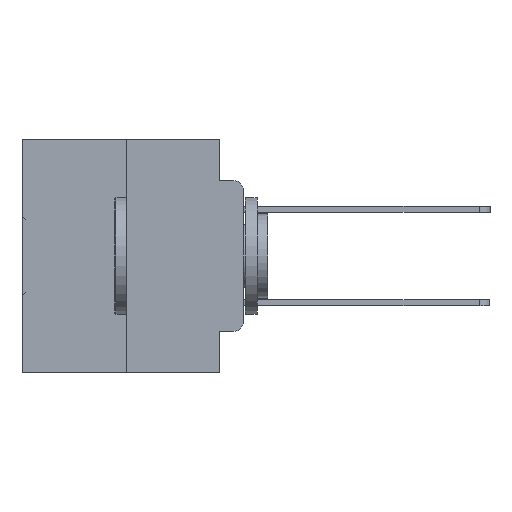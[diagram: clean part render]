
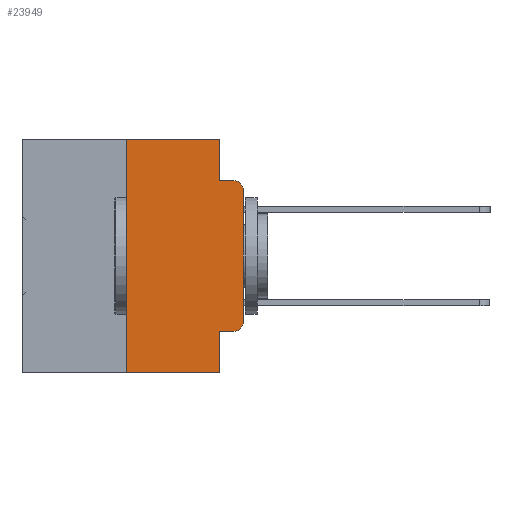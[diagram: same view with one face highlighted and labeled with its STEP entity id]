
A CAD part, left-side view. The second image highlights one B-rep face of the part: STEP entity #23949.
In plain terms, the highlighted planar face has unit normal (-1, 0, 0).
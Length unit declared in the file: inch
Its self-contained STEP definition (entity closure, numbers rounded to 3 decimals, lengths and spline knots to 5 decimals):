
#451 = CARTESIAN_POINT ( 'NONE',  ( 0., 0.25, 0. ) ) ;
#971 = CARTESIAN_POINT ( 'NONE',  ( 0., 0., 0. ) ) ;
#1278 = CARTESIAN_POINT ( 'NONE',  ( 0., 0.473, -0.5 ) ) ;
#2101 = CARTESIAN_POINT ( 'NONE',  ( 0., 0.051, 0. ) ) ;
#2289 = AXIS2_PLACEMENT_3D ( 'NONE', #9709, #33688, #33618 ) ;
#3252 = VERTEX_POINT ( 'NONE', #20303 ) ;
#3353 = EDGE_CURVE ( 'NONE', #3252, #34849, #17456, .T. ) ;
#3633 = VERTEX_POINT ( 'NONE', #451 ) ;
#3754 = DIRECTION ( 'NONE',  ( 0., 0., 1. ) ) ;
#3814 = EDGE_CURVE ( 'NONE', #25659, #6525, #9236, .T. ) ;
#3856 = CARTESIAN_POINT ( 'NONE',  ( 0., 0.473, 0. ) ) ;
#3918 = VECTOR ( 'NONE', #20475, 39.37008 ) ;
#4175 = LINE ( 'NONE', #971, #11537 ) ;
#4646 = ORIENTED_EDGE ( 'NONE', *, *, #3814, .T. ) ;
#4874 = DIRECTION ( 'NONE',  ( 0., 0., -1. ) ) ;
#4879 = VERTEX_POINT ( 'NONE', #22908 ) ;
#5162 = LINE ( 'NONE', #27346, #18997 ) ;
#6348 = EDGE_CURVE ( 'NONE', #4879, #3633, #18604, .T. ) ;
#6525 = VERTEX_POINT ( 'NONE', #30867 ) ;
#6730 = DIRECTION ( 'NONE',  ( 0., -1., 0. ) ) ;
#6808 = DIRECTION ( 'NONE',  ( 0., -1., 0. ) ) ;
#7438 = CARTESIAN_POINT ( 'NONE',  ( 0., 0.051, 0. ) ) ;
#7561 = DIRECTION ( 'NONE',  ( 0., 0., -1. ) ) ;
#7734 = CARTESIAN_POINT ( 'NONE',  ( 0., 0.051, -0.0885 ) ) ;
#7760 = EDGE_CURVE ( 'NONE', #4879, #29713, #17618, .T. ) ;
#8117 = ORIENTED_EDGE ( 'NONE', *, *, #13785, .F. ) ;
#8230 = CARTESIAN_POINT ( 'NONE',  ( 0., 0.473, 0. ) ) ;
#9067 = VECTOR ( 'NONE', #6730, 39.37008 ) ;
#9236 = CIRCLE ( 'NONE', #18238, 0.02 ) ;
#9709 = CARTESIAN_POINT ( 'NONE',  ( 0., 0.02, -0.3915 ) ) ;
#9847 = ORIENTED_EDGE ( 'NONE', *, *, #22464, .F. ) ;
#10311 = ORIENTED_EDGE ( 'NONE', *, *, #3353, .T. ) ;
#10497 = CARTESIAN_POINT ( 'NONE',  ( 0., 0., -0.3915 ) ) ;
#10728 = VECTOR ( 'NONE', #4874, 39.37008 ) ;
#11012 = DIRECTION ( 'NONE',  ( 0., 0., -1. ) ) ;
#11384 = CARTESIAN_POINT ( 'NONE',  ( 0., 0.051, 0. ) ) ;
#11405 = DIRECTION ( 'NONE',  ( 0., 0., -1. ) ) ;
#11452 = DIRECTION ( 'NONE',  ( -1., 0., 0. ) ) ;
#11457 = CARTESIAN_POINT ( 'NONE',  ( 0., 0.02, -0.1085 ) ) ;
#11537 = VECTOR ( 'NONE', #3754, 39.37008 ) ;
#11588 = ORIENTED_EDGE ( 'NONE', *, *, #6348, .F. ) ;
#11998 = VECTOR ( 'NONE', #7561, 39.37008 ) ;
#12059 = AXIS2_PLACEMENT_3D ( 'NONE', #8230, #27543, #11012 ) ;
#12617 = EDGE_CURVE ( 'NONE', #27718, #3252, #5162, .T. ) ;
#13785 = EDGE_CURVE ( 'NONE', #29463, #30838, #26687, .T. ) ;
#14989 = CARTESIAN_POINT ( 'NONE',  ( 0., 0.051, -0.5 ) ) ;
#15268 = LINE ( 'NONE', #24024, #22658 ) ;
#17016 = CARTESIAN_POINT ( 'NONE',  ( 0., 0.051, -0.4115 ) ) ;
#17244 = LINE ( 'NONE', #3856, #9067 ) ;
#17456 = CIRCLE ( 'NONE', #2289, 0.02 ) ;
#17618 = LINE ( 'NONE', #1278, #29750 ) ;
#18238 = AXIS2_PLACEMENT_3D ( 'NONE', #11457, #11452, #11405 ) ;
#18467 = ORIENTED_EDGE ( 'NONE', *, *, #24202, .T. ) ;
#18604 = LINE ( 'NONE', #28901, #3918 ) ;
#18997 = VECTOR ( 'NONE', #24615, 39.37008 ) ;
#19333 = EDGE_CURVE ( 'NONE', #30838, #6525, #15268, .T. ) ;
#19432 = CARTESIAN_POINT ( 'NONE',  ( 0., 0., -0.1085 ) ) ;
#20303 = CARTESIAN_POINT ( 'NONE',  ( 0., 0.02, -0.4115 ) ) ;
#20475 = DIRECTION ( 'NONE',  ( 0., 0., 1. ) ) ;
#20651 = ORIENTED_EDGE ( 'NONE', *, *, #29250, .F. ) ;
#21728 = EDGE_LOOP ( 'NONE', ( #18467, #4646, #34809, #8117, #9847, #11588, #33573, #20651, #29746, #10311 ) ) ;
#22031 = PLANE ( 'NONE',  #12059 ) ;
#22464 = EDGE_CURVE ( 'NONE', #3633, #29463, #17244, .T. ) ;
#22658 = VECTOR ( 'NONE', #23896, 39.37008 ) ;
#22908 = CARTESIAN_POINT ( 'NONE',  ( 0., 0.25, -0.5 ) ) ;
#23896 = DIRECTION ( 'NONE',  ( 0., -1., 0. ) ) ;
#23949 = ADVANCED_FACE ( 'NONE', ( #24975 ), #22031, .F. ) ;
#24024 = CARTESIAN_POINT ( 'NONE',  ( 0., 0.051, -0.0885 ) ) ;
#24202 = EDGE_CURVE ( 'NONE', #34849, #25659, #4175, .T. ) ;
#24615 = DIRECTION ( 'NONE',  ( 0., -1., 0. ) ) ;
#24975 = FACE_OUTER_BOUND ( 'NONE', #21728, .T. ) ;
#25659 = VERTEX_POINT ( 'NONE', #19432 ) ;
#26687 = LINE ( 'NONE', #7438, #11998 ) ;
#27346 = CARTESIAN_POINT ( 'NONE',  ( 0., 0.051, -0.4115 ) ) ;
#27543 = DIRECTION ( 'NONE',  ( 1., 0., 0. ) ) ;
#27718 = VERTEX_POINT ( 'NONE', #17016 ) ;
#28901 = CARTESIAN_POINT ( 'NONE',  ( 0., 0.25, 0. ) ) ;
#29250 = EDGE_CURVE ( 'NONE', #27718, #29713, #32726, .T. ) ;
#29463 = VERTEX_POINT ( 'NONE', #11384 ) ;
#29713 = VERTEX_POINT ( 'NONE', #14989 ) ;
#29746 = ORIENTED_EDGE ( 'NONE', *, *, #12617, .T. ) ;
#29750 = VECTOR ( 'NONE', #6808, 39.37008 ) ;
#30838 = VERTEX_POINT ( 'NONE', #7734 ) ;
#30867 = CARTESIAN_POINT ( 'NONE',  ( 0., 0.02, -0.0885 ) ) ;
#32726 = LINE ( 'NONE', #2101, #10728 ) ;
#33573 = ORIENTED_EDGE ( 'NONE', *, *, #7760, .T. ) ;
#33618 = DIRECTION ( 'NONE',  ( 0., 0., -1. ) ) ;
#33688 = DIRECTION ( 'NONE',  ( -1., 0., 0. ) ) ;
#34809 = ORIENTED_EDGE ( 'NONE', *, *, #19333, .F. ) ;
#34849 = VERTEX_POINT ( 'NONE', #10497 ) ;
